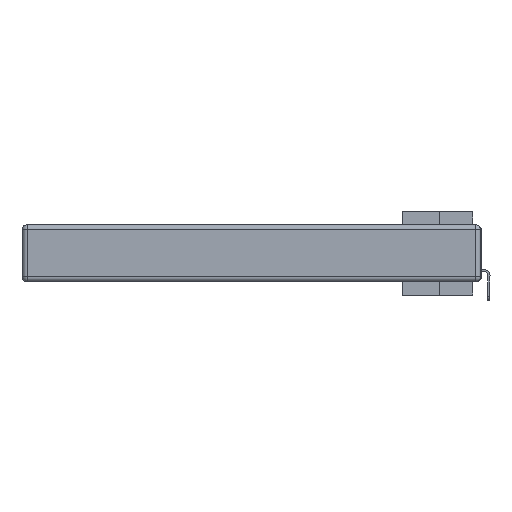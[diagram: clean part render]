
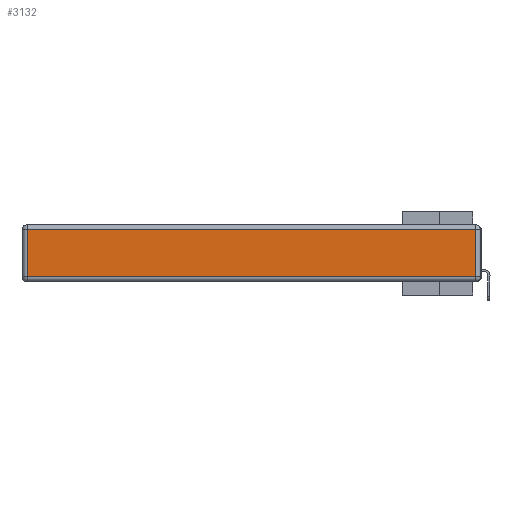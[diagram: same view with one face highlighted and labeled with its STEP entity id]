
A CAD part, left-side view. The second image highlights one B-rep face of the part: STEP entity #3132.
In plain terms, the highlighted planar face has unit normal (-1, 0, 0).
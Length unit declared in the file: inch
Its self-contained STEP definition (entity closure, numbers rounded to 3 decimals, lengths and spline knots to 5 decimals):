
#1151 = VECTOR ( 'NONE', #7720, 39.37008 ) ;
#2394 = VERTEX_POINT ( 'NONE', #6719 ) ;
#3132 = ADVANCED_FACE ( 'NONE', ( #5025 ), #33889, .T. ) ;
#5025 = FACE_OUTER_BOUND ( 'NONE', #7426, .T. ) ;
#5173 = EDGE_CURVE ( 'NONE', #5293, #2394, #16793, .T. ) ;
#5293 = VERTEX_POINT ( 'NONE', #20143 ) ;
#5937 = CARTESIAN_POINT ( 'NONE',  ( 0., 0., -0.313 ) ) ;
#6719 = CARTESIAN_POINT ( 'NONE',  ( 0., 0.03, -0.03 ) ) ;
#7426 = EDGE_LOOP ( 'NONE', ( #36080, #18846, #19686, #12301 ) ) ;
#7720 = DIRECTION ( 'NONE',  ( 0., 1., 0. ) ) ;
#11978 = CARTESIAN_POINT ( 'NONE',  ( 0., 0., -0.343 ) ) ;
#12301 = ORIENTED_EDGE ( 'NONE', *, *, #34546, .T. ) ;
#13002 = DIRECTION ( 'NONE',  ( 0., 0., -1. ) ) ;
#14606 = CARTESIAN_POINT ( 'NONE',  ( 0., 2.72, -0.03 ) ) ;
#16793 = LINE ( 'NONE', #31822, #35661 ) ;
#17903 = VERTEX_POINT ( 'NONE', #14606 ) ;
#18513 = EDGE_CURVE ( 'NONE', #23166, #5293, #35971, .T. ) ;
#18846 = ORIENTED_EDGE ( 'NONE', *, *, #5173, .T. ) ;
#18878 = EDGE_CURVE ( 'NONE', #2394, #17903, #39352, .T. ) ;
#19411 = AXIS2_PLACEMENT_3D ( 'NONE', #11978, #30574, #30846 ) ;
#19686 = ORIENTED_EDGE ( 'NONE', *, *, #18878, .T. ) ;
#20143 = CARTESIAN_POINT ( 'NONE',  ( 0., 0.03, -0.313 ) ) ;
#23166 = VERTEX_POINT ( 'NONE', #25819 ) ;
#25588 = CARTESIAN_POINT ( 'NONE',  ( 0., 2.72, -0.343 ) ) ;
#25819 = CARTESIAN_POINT ( 'NONE',  ( 0., 2.72, -0.313 ) ) ;
#25976 = VECTOR ( 'NONE', #40324, 39.37008 ) ;
#27200 = LINE ( 'NONE', #25588, #35660 ) ;
#30574 = DIRECTION ( 'NONE',  ( -1., 0., 0. ) ) ;
#30846 = DIRECTION ( 'NONE',  ( 0., 0., 1. ) ) ;
#31822 = CARTESIAN_POINT ( 'NONE',  ( 0., 0.03, -0.343 ) ) ;
#31961 = DIRECTION ( 'NONE',  ( 0., 0., 1. ) ) ;
#33889 = PLANE ( 'NONE',  #19411 ) ;
#34546 = EDGE_CURVE ( 'NONE', #17903, #23166, #27200, .T. ) ;
#35660 = VECTOR ( 'NONE', #13002, 39.37008 ) ;
#35661 = VECTOR ( 'NONE', #31961, 39.37008 ) ;
#35971 = LINE ( 'NONE', #5937, #25976 ) ;
#36080 = ORIENTED_EDGE ( 'NONE', *, *, #18513, .T. ) ;
#39352 = LINE ( 'NONE', #39453, #1151 ) ;
#39453 = CARTESIAN_POINT ( 'NONE',  ( 0., 2.75, -0.03 ) ) ;
#40324 = DIRECTION ( 'NONE',  ( 0., -1., 0. ) ) ;
